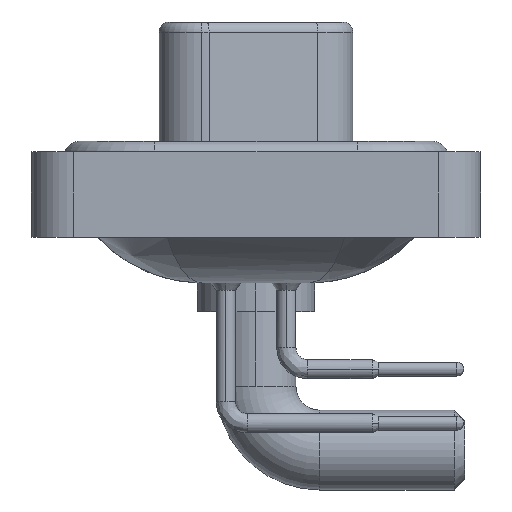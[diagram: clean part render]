
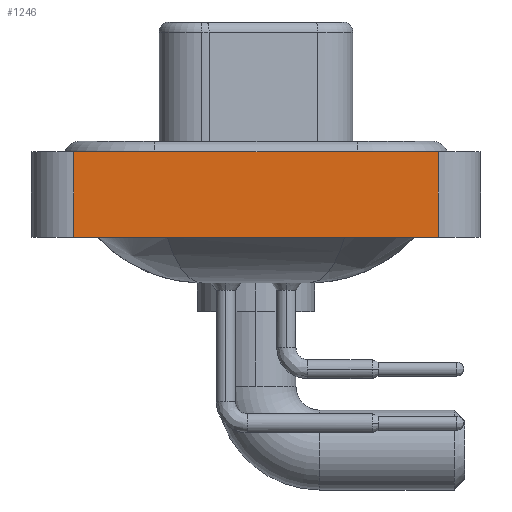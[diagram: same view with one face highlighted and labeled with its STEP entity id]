
A CAD part, left-side view. The second image highlights one B-rep face of the part: STEP entity #1246.
In plain terms, the highlighted planar face has unit normal (-1, 0, 0).
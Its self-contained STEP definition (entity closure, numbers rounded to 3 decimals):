
#485 = CARTESIAN_POINT ( 'NONE',  ( -7.3, 8.55, 0.4 ) ) ;
#1114 = VECTOR ( 'NONE', #20043, 1000. ) ;
#1246 = ADVANCED_FACE ( 'NONE', ( #4995 ), #14994, .T. ) ;
#1586 = CARTESIAN_POINT ( 'NONE',  ( -7.3, -8.55, 0.4 ) ) ;
#1869 = ORIENTED_EDGE ( 'NONE', *, *, #7462, .T. ) ;
#2114 = CARTESIAN_POINT ( 'NONE',  ( -7.3, 8.55, -3.6 ) ) ;
#3028 = CARTESIAN_POINT ( 'NONE',  ( -7.3, -8.55, 0.4 ) ) ;
#3777 = DIRECTION ( 'NONE',  ( 0., 0., 1. ) ) ;
#4013 = CARTESIAN_POINT ( 'NONE',  ( -7.3, -8.55, -3.6 ) ) ;
#4995 = FACE_OUTER_BOUND ( 'NONE', #15122, .T. ) ;
#5796 = EDGE_CURVE ( 'NONE', #10100, #10842, #18120, .T. ) ;
#7462 = EDGE_CURVE ( 'NONE', #18518, #10100, #12005, .T. ) ;
#7476 = LINE ( 'NONE', #3028, #24139 ) ;
#8872 = AXIS2_PLACEMENT_3D ( 'NONE', #12667, #12788, #10553 ) ;
#9817 = DIRECTION ( 'NONE',  ( 0., 0., 1. ) ) ;
#10100 = VERTEX_POINT ( 'NONE', #22573 ) ;
#10553 = DIRECTION ( 'NONE',  ( 0., 0., 1. ) ) ;
#10842 = VERTEX_POINT ( 'NONE', #1586 ) ;
#12005 = LINE ( 'NONE', #16592, #1114 ) ;
#12667 = CARTESIAN_POINT ( 'NONE',  ( -7.3, -8.55, -3.6 ) ) ;
#12788 = DIRECTION ( 'NONE',  ( -1., 0., 0. ) ) ;
#14513 = ORIENTED_EDGE ( 'NONE', *, *, #5796, .T. ) ;
#14872 = VECTOR ( 'NONE', #3777, 1000. ) ;
#14994 = PLANE ( 'NONE',  #8872 ) ;
#15122 = EDGE_LOOP ( 'NONE', ( #14513, #22711, #21223, #1869 ) ) ;
#16592 = CARTESIAN_POINT ( 'NONE',  ( -7.3, -8.55, -3.6 ) ) ;
#17252 = DIRECTION ( 'NONE',  ( 0., -1., 0. ) ) ;
#17527 = EDGE_CURVE ( 'NONE', #18518, #19883, #17615, .T. ) ;
#17615 = LINE ( 'NONE', #23417, #14872 ) ;
#18120 = LINE ( 'NONE', #4013, #23530 ) ;
#18518 = VERTEX_POINT ( 'NONE', #2114 ) ;
#19883 = VERTEX_POINT ( 'NONE', #485 ) ;
#20043 = DIRECTION ( 'NONE',  ( 0., -1., 0. ) ) ;
#21030 = EDGE_CURVE ( 'NONE', #19883, #10842, #7476, .T. ) ;
#21223 = ORIENTED_EDGE ( 'NONE', *, *, #17527, .F. ) ;
#22573 = CARTESIAN_POINT ( 'NONE',  ( -7.3, -8.55, -3.6 ) ) ;
#22711 = ORIENTED_EDGE ( 'NONE', *, *, #21030, .F. ) ;
#23417 = CARTESIAN_POINT ( 'NONE',  ( -7.3, 8.55, -3.6 ) ) ;
#23530 = VECTOR ( 'NONE', #9817, 1000. ) ;
#24139 = VECTOR ( 'NONE', #17252, 1000. ) ;
